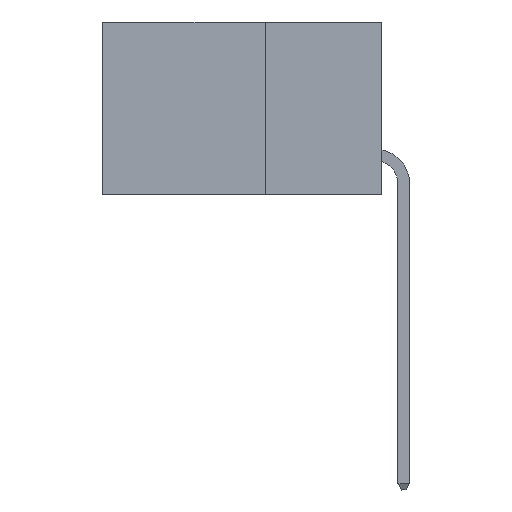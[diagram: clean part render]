
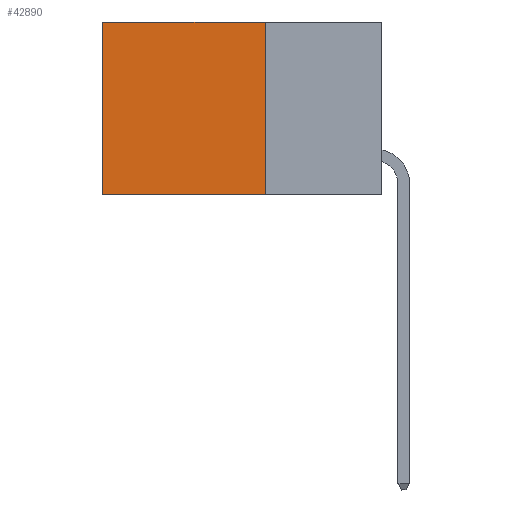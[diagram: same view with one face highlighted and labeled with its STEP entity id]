
A CAD part, left-side view. The second image highlights one B-rep face of the part: STEP entity #42890.
In plain terms, the highlighted planar face has unit normal (-1, 0, 0).
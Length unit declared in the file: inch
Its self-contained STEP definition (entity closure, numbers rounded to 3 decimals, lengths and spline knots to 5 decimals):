
#134 = ORIENTED_EDGE ( 'NONE', *, *, #5697, .F. ) ;
#558 = VECTOR ( 'NONE', #38050, 39.37008 ) ;
#1480 = VERTEX_POINT ( 'NONE', #25360 ) ;
#3375 = CARTESIAN_POINT ( 'NONE',  ( 0.2875, 0.25, 0. ) ) ;
#3881 = LINE ( 'NONE', #44707, #558 ) ;
#5697 = EDGE_CURVE ( 'NONE', #8711, #1480, #3881, .T. ) ;
#6256 = LINE ( 'NONE', #30597, #10046 ) ;
#6854 = CARTESIAN_POINT ( 'NONE',  ( 0.2875, 0.6, 0. ) ) ;
#6858 = ORIENTED_EDGE ( 'NONE', *, *, #29841, .F. ) ;
#8711 = VERTEX_POINT ( 'NONE', #27049 ) ;
#9527 = DIRECTION ( 'NONE',  ( 1., 0., 0. ) ) ;
#9832 = PLANE ( 'NONE',  #16209 ) ;
#10046 = VECTOR ( 'NONE', #41392, 39.37008 ) ;
#10058 = EDGE_CURVE ( 'NONE', #38270, #1480, #35284, .T. ) ;
#16209 = AXIS2_PLACEMENT_3D ( 'NONE', #23303, #9527, #27171 ) ;
#16502 = CARTESIAN_POINT ( 'NONE',  ( 0.2875, 0.6, 0. ) ) ;
#18204 = FACE_OUTER_BOUND ( 'NONE', #24584, .T. ) ;
#19355 = DIRECTION ( 'NONE',  ( 0., 0., -1. ) ) ;
#20480 = ORIENTED_EDGE ( 'NONE', *, *, #34020, .T. ) ;
#21488 = VERTEX_POINT ( 'NONE', #33970 ) ;
#23303 = CARTESIAN_POINT ( 'NONE',  ( 0.2875, 0.25, 0. ) ) ;
#24584 = EDGE_LOOP ( 'NONE', ( #36805, #134, #6858, #20480 ) ) ;
#25360 = CARTESIAN_POINT ( 'NONE',  ( 0.2875, 0.6, -0.37 ) ) ;
#27049 = CARTESIAN_POINT ( 'NONE',  ( 0.2875, 0.25, -0.37 ) ) ;
#27088 = VECTOR ( 'NONE', #19355, 39.37008 ) ;
#27171 = DIRECTION ( 'NONE',  ( 0., 0., -1. ) ) ;
#27902 = DIRECTION ( 'NONE',  ( 0., 0., -1. ) ) ;
#29841 = EDGE_CURVE ( 'NONE', #21488, #8711, #33040, .T. ) ;
#30597 = CARTESIAN_POINT ( 'NONE',  ( 0.2875, 0.25, 0. ) ) ;
#33040 = LINE ( 'NONE', #3375, #38976 ) ;
#33970 = CARTESIAN_POINT ( 'NONE',  ( 0.2875, 0.25, 0. ) ) ;
#34020 = EDGE_CURVE ( 'NONE', #21488, #38270, #6256, .T. ) ;
#35284 = LINE ( 'NONE', #16502, #27088 ) ;
#36805 = ORIENTED_EDGE ( 'NONE', *, *, #10058, .T. ) ;
#38050 = DIRECTION ( 'NONE',  ( 0., 1., 0. ) ) ;
#38270 = VERTEX_POINT ( 'NONE', #6854 ) ;
#38976 = VECTOR ( 'NONE', #27902, 39.37008 ) ;
#41392 = DIRECTION ( 'NONE',  ( 0., 1., 0. ) ) ;
#42890 = ADVANCED_FACE ( 'NONE', ( #18204 ), #9832, .F. ) ;
#44707 = CARTESIAN_POINT ( 'NONE',  ( 0.2875, 0.25, -0.37 ) ) ;
